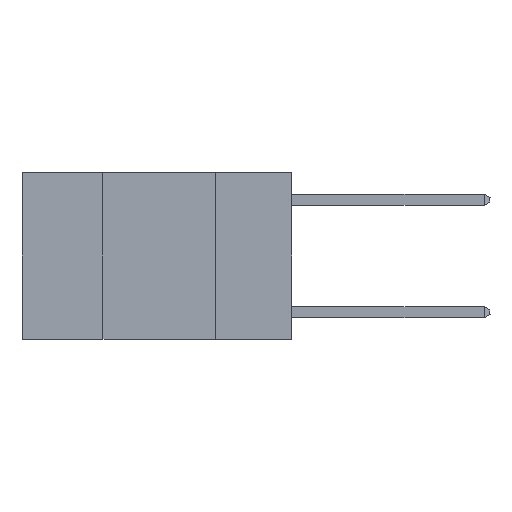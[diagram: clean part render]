
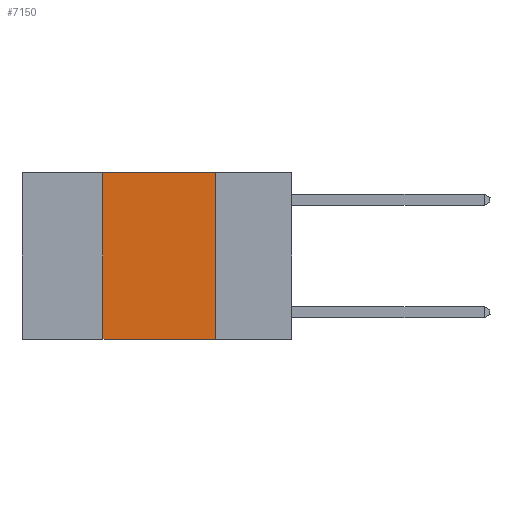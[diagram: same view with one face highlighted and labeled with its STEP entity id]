
A CAD part, left-side view. The second image highlights one B-rep face of the part: STEP entity #7150.
In plain terms, the highlighted planar face has unit normal (-1, 0, 0).
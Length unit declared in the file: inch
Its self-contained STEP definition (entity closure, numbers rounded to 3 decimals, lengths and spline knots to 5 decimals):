
#118 = CARTESIAN_POINT ( 'NONE',  ( 0., 0.17, 0. ) ) ;
#1955 = DIRECTION ( 'NONE',  ( 1., 0., 0. ) ) ;
#2405 = EDGE_CURVE ( 'NONE', #7254, #3875, #14887, .T. ) ;
#3072 = VECTOR ( 'NONE', #17656, 39.37008 ) ;
#3178 = CARTESIAN_POINT ( 'NONE',  ( 0., 0.6, 0. ) ) ;
#3285 = CARTESIAN_POINT ( 'NONE',  ( 0., 0.42, -0.37 ) ) ;
#3875 = VERTEX_POINT ( 'NONE', #13324 ) ;
#3980 = LINE ( 'NONE', #118, #14791 ) ;
#5790 = ORIENTED_EDGE ( 'NONE', *, *, #20157, .F. ) ;
#7150 = ADVANCED_FACE ( 'NONE', ( #12001 ), #23962, .F. ) ;
#7254 = VERTEX_POINT ( 'NONE', #25113 ) ;
#8098 = ORIENTED_EDGE ( 'NONE', *, *, #2405, .F. ) ;
#8188 = VERTEX_POINT ( 'NONE', #8954 ) ;
#8954 = CARTESIAN_POINT ( 'NONE',  ( 0., 0.17, -0.37 ) ) ;
#9908 = DIRECTION ( 'NONE',  ( 0., 0., 1. ) ) ;
#11703 = VECTOR ( 'NONE', #9908, 39.37008 ) ;
#11950 = DIRECTION ( 'NONE',  ( 0., 0., -1. ) ) ;
#12001 = FACE_OUTER_BOUND ( 'NONE', #13456, .T. ) ;
#13324 = CARTESIAN_POINT ( 'NONE',  ( 0., 0.17, 0. ) ) ;
#13456 = EDGE_LOOP ( 'NONE', ( #14979, #8098, #5790, #14742 ) ) ;
#13806 = LINE ( 'NONE', #17041, #3072 ) ;
#14742 = ORIENTED_EDGE ( 'NONE', *, *, #20059, .T. ) ;
#14791 = VECTOR ( 'NONE', #11950, 39.37008 ) ;
#14887 = LINE ( 'NONE', #3178, #16539 ) ;
#14979 = ORIENTED_EDGE ( 'NONE', *, *, #24120, .F. ) ;
#15977 = LINE ( 'NONE', #19710, #11703 ) ;
#16539 = VECTOR ( 'NONE', #18872, 39.37008 ) ;
#17041 = CARTESIAN_POINT ( 'NONE',  ( 0., 0.6, -0.37 ) ) ;
#17656 = DIRECTION ( 'NONE',  ( 0., -1., 0. ) ) ;
#18055 = DIRECTION ( 'NONE',  ( 0., 0., -1. ) ) ;
#18872 = DIRECTION ( 'NONE',  ( 0., -1., 0. ) ) ;
#19710 = CARTESIAN_POINT ( 'NONE',  ( 0., 0.42, 0. ) ) ;
#20059 = EDGE_CURVE ( 'NONE', #25257, #8188, #13806, .T. ) ;
#20157 = EDGE_CURVE ( 'NONE', #25257, #7254, #15977, .T. ) ;
#21662 = CARTESIAN_POINT ( 'NONE',  ( 0., 0.6, 0. ) ) ;
#23142 = AXIS2_PLACEMENT_3D ( 'NONE', #21662, #1955, #18055 ) ;
#23962 = PLANE ( 'NONE',  #23142 ) ;
#24120 = EDGE_CURVE ( 'NONE', #3875, #8188, #3980, .T. ) ;
#25113 = CARTESIAN_POINT ( 'NONE',  ( 0., 0.42, 0. ) ) ;
#25257 = VERTEX_POINT ( 'NONE', #3285 ) ;
